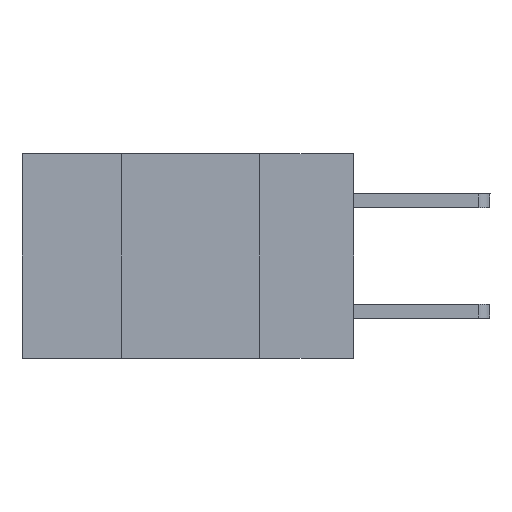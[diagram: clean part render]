
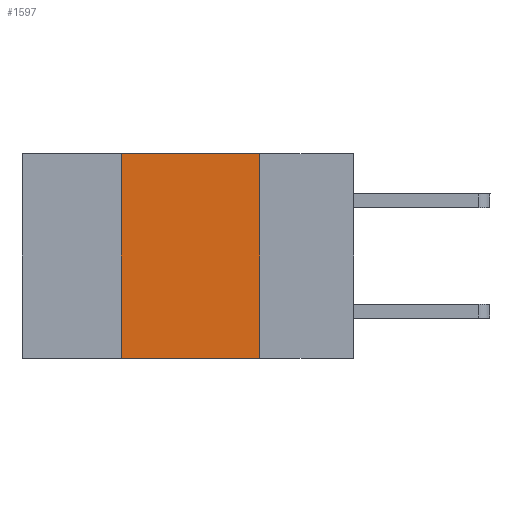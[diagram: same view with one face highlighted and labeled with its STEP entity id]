
A CAD part, left-side view. The second image highlights one B-rep face of the part: STEP entity #1597.
In plain terms, the highlighted planar face has unit normal (-1, 0, 0).
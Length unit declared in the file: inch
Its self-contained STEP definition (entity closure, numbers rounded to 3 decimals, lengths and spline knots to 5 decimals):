
#89 = EDGE_LOOP ( 'NONE', ( #1622, #7556, #3591, #221 ) ) ;
#221 = ORIENTED_EDGE ( 'NONE', *, *, #4084, .T. ) ;
#502 = LINE ( 'NONE', #6435, #908 ) ;
#793 = CARTESIAN_POINT ( 'NONE',  ( 0., 0.17, -0.37 ) ) ;
#908 = VECTOR ( 'NONE', #6728, 39.37008 ) ;
#994 = FACE_OUTER_BOUND ( 'NONE', #89, .T. ) ;
#1597 = ADVANCED_FACE ( 'NONE', ( #994 ), #11450, .F. ) ;
#1622 = ORIENTED_EDGE ( 'NONE', *, *, #4920, .F. ) ;
#2002 = CARTESIAN_POINT ( 'NONE',  ( 0., 0.6, -0.37 ) ) ;
#2124 = LINE ( 'NONE', #10758, #3622 ) ;
#2240 = VERTEX_POINT ( 'NONE', #793 ) ;
#2304 = CARTESIAN_POINT ( 'NONE',  ( 0., 0.17, 0. ) ) ;
#2646 = VERTEX_POINT ( 'NONE', #2304 ) ;
#2925 = EDGE_CURVE ( 'NONE', #6478, #6930, #7958, .T. ) ;
#3528 = CARTESIAN_POINT ( 'NONE',  ( 0., 0.42, -0.37 ) ) ;
#3591 = ORIENTED_EDGE ( 'NONE', *, *, #2925, .F. ) ;
#3622 = VECTOR ( 'NONE', #9889, 39.37008 ) ;
#3943 = AXIS2_PLACEMENT_3D ( 'NONE', #8996, #7248, #3983 ) ;
#3983 = DIRECTION ( 'NONE',  ( 0., 0., -1. ) ) ;
#4084 = EDGE_CURVE ( 'NONE', #6478, #2240, #6262, .T. ) ;
#4645 = VECTOR ( 'NONE', #5546, 39.37008 ) ;
#4920 = EDGE_CURVE ( 'NONE', #2646, #2240, #502, .T. ) ;
#4922 = CARTESIAN_POINT ( 'NONE',  ( 0., 0.42, 0. ) ) ;
#5546 = DIRECTION ( 'NONE',  ( 0., -1., 0. ) ) ;
#5850 = CARTESIAN_POINT ( 'NONE',  ( 0., 0.42, 0. ) ) ;
#6262 = LINE ( 'NONE', #2002, #4645 ) ;
#6435 = CARTESIAN_POINT ( 'NONE',  ( 0., 0.17, 0. ) ) ;
#6478 = VERTEX_POINT ( 'NONE', #3528 ) ;
#6728 = DIRECTION ( 'NONE',  ( 0., 0., -1. ) ) ;
#6930 = VERTEX_POINT ( 'NONE', #4922 ) ;
#7248 = DIRECTION ( 'NONE',  ( 1., 0., 0. ) ) ;
#7556 = ORIENTED_EDGE ( 'NONE', *, *, #9012, .F. ) ;
#7958 = LINE ( 'NONE', #5850, #11052 ) ;
#8996 = CARTESIAN_POINT ( 'NONE',  ( 0., 0.6, 0. ) ) ;
#9012 = EDGE_CURVE ( 'NONE', #6930, #2646, #2124, .T. ) ;
#9889 = DIRECTION ( 'NONE',  ( 0., -1., 0. ) ) ;
#10327 = DIRECTION ( 'NONE',  ( 0., 0., 1. ) ) ;
#10758 = CARTESIAN_POINT ( 'NONE',  ( 0., 0.6, 0. ) ) ;
#11052 = VECTOR ( 'NONE', #10327, 39.37008 ) ;
#11450 = PLANE ( 'NONE',  #3943 ) ;
